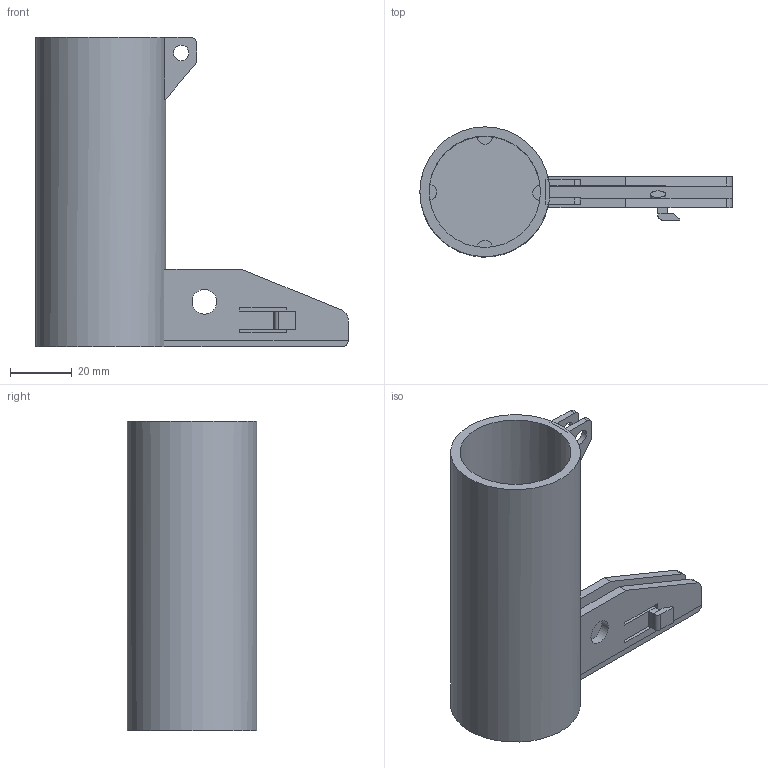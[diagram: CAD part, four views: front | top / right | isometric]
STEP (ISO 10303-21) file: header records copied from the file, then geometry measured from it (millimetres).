
FILE_DESCRIPTION(('FreeCAD Model'),'2;1');
FILE_NAME('ap9 folding arm brace tube 2020.step','2020-04-04T17:46:12',('Author'),(''), 'Open CASCADE STEP processor 6.8','FreeCAD','Unknown');
FILE_SCHEMA(('AUTOMOTIVE_DESIGN_CC2 { 1 2 10303 214 -1 1 5 4 }'));
Length unit declared in the file: millimetre
Products named in the file (1): Fillet003
Bounding box: 101 x 42 x 100 mm (x, y, z)
Volume: 48365.2 mm3; surface area: 33734.5 mm2
Topology: 1 solids, 1 shells, 84 faces, 220 edges, 140 vertices
Faces by surface type: plane 62, cylinder 22
Full cylindrical faces by diameter (mm): 5 x3, 8 x2, 36 x1, 42 x1
Entity records: 5565 total; most frequent: CARTESIAN_POINT 1260, DIRECTION 778, LINE 451, VECTOR 451, ORIENTED_EDGE 440, PCURVE 440, DEFINITIONAL_REPRESENTATION 440, EDGE_CURVE 220
